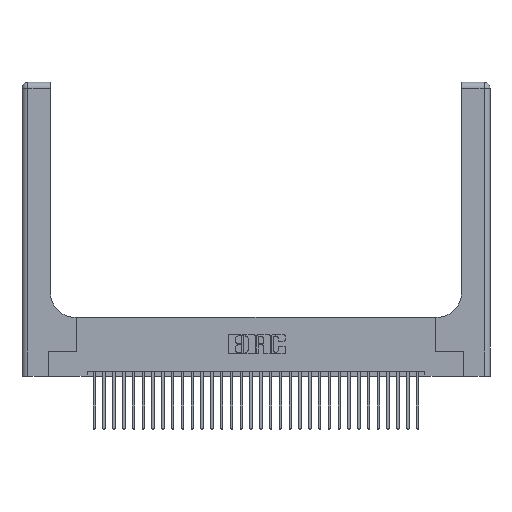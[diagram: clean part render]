
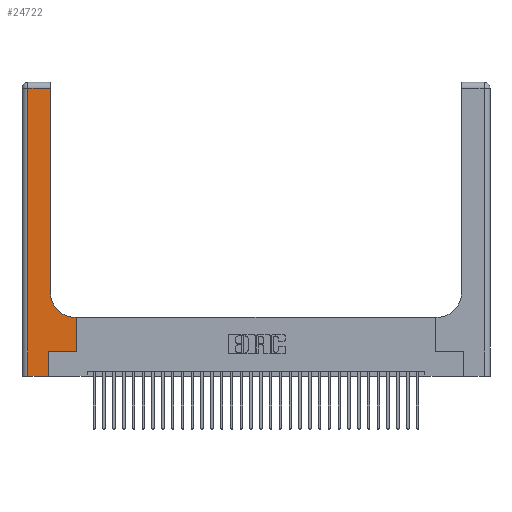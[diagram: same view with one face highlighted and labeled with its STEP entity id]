
A CAD part, top view. The second image highlights one B-rep face of the part: STEP entity #24722.
In plain terms, the highlighted planar face has unit normal (0, 0, 1).
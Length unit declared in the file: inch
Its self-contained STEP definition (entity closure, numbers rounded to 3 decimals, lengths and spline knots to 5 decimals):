
#365 = DIRECTION ( 'NONE',  ( -1., 0., 0. ) ) ;
#416 = VERTEX_POINT ( 'NONE', #21749 ) ;
#425 = EDGE_CURVE ( 'NONE', #14012, #24214, #13060, .T. ) ;
#596 = CARTESIAN_POINT ( 'NONE',  ( 0.5585, 0.25, 0.37 ) ) ;
#1376 = DIRECTION ( 'NONE',  ( -1., 0., 0. ) ) ;
#1511 = DIRECTION ( 'NONE',  ( 0., 1., 0. ) ) ;
#1523 = VERTEX_POINT ( 'NONE', #18330 ) ;
#1791 = VERTEX_POINT ( 'NONE', #2879 ) ;
#1811 = PLANE ( 'NONE',  #15789 ) ;
#2296 = VECTOR ( 'NONE', #27304, 39.37008 ) ;
#2879 = CARTESIAN_POINT ( 'NONE',  ( 0.269, 0., 0.37 ) ) ;
#2910 = EDGE_CURVE ( 'NONE', #24214, #5168, #25202, .T. ) ;
#3036 = FACE_OUTER_BOUND ( 'NONE', #20040, .T. ) ;
#3267 = CARTESIAN_POINT ( 'NONE',  ( 0.2915, 0.6, 0.37 ) ) ;
#4148 = CARTESIAN_POINT ( 'NONE',  ( 0., 3., 0.37 ) ) ;
#4423 = ORIENTED_EDGE ( 'NONE', *, *, #25913, .T. ) ;
#4759 = VECTOR ( 'NONE', #365, 39.37008 ) ;
#4827 = CARTESIAN_POINT ( 'NONE',  ( 0.06, 3., 0.37 ) ) ;
#5168 = VERTEX_POINT ( 'NONE', #31244 ) ;
#5522 = LINE ( 'NONE', #3267, #4759 ) ;
#6485 = CARTESIAN_POINT ( 'NONE',  ( 0.269, 0., 0.37 ) ) ;
#6946 = DIRECTION ( 'NONE',  ( 0., 0., -1. ) ) ;
#7225 = ORIENTED_EDGE ( 'NONE', *, *, #2910, .T. ) ;
#7393 = VECTOR ( 'NONE', #1511, 39.37008 ) ;
#7637 = CARTESIAN_POINT ( 'NONE',  ( 0., 0., 0.37 ) ) ;
#8522 = ORIENTED_EDGE ( 'NONE', *, *, #13523, .T. ) ;
#9076 = LINE ( 'NONE', #4827, #2296 ) ;
#9841 = LINE ( 'NONE', #21091, #22919 ) ;
#10006 = ORIENTED_EDGE ( 'NONE', *, *, #32723, .T. ) ;
#12406 = EDGE_CURVE ( 'NONE', #32494, #1523, #5522, .T. ) ;
#13060 = LINE ( 'NONE', #26183, #21402 ) ;
#13523 = EDGE_CURVE ( 'NONE', #5168, #26957, #9076, .T. ) ;
#14012 = VERTEX_POINT ( 'NONE', #28362 ) ;
#14065 = CARTESIAN_POINT ( 'NONE',  ( 0., 2.94, 0.37 ) ) ;
#14221 = DIRECTION ( 'NONE',  ( 1., 0., 0. ) ) ;
#15660 = CARTESIAN_POINT ( 'NONE',  ( 0.5585, 0.6, 0.37 ) ) ;
#15771 = VECTOR ( 'NONE', #23073, 39.37008 ) ;
#15789 = AXIS2_PLACEMENT_3D ( 'NONE', #4148, #32531, #19556 ) ;
#16133 = LINE ( 'NONE', #25100, #24888 ) ;
#16143 = ORIENTED_EDGE ( 'NONE', *, *, #12406, .T. ) ;
#16221 = DIRECTION ( 'NONE',  ( 0., 1., 0. ) ) ;
#17216 = EDGE_CURVE ( 'NONE', #20277, #32494, #9841, .T. ) ;
#17591 = CARTESIAN_POINT ( 'NONE',  ( 0.2915, 2.94, 0.37 ) ) ;
#17864 = EDGE_CURVE ( 'NONE', #416, #20277, #16133, .T. ) ;
#18121 = LINE ( 'NONE', #6485, #7393 ) ;
#18330 = CARTESIAN_POINT ( 'NONE',  ( 0.5415, 0.6, 0.37 ) ) ;
#19230 = VECTOR ( 'NONE', #1376, 39.37008 ) ;
#19556 = DIRECTION ( 'NONE',  ( -1., 0., 0. ) ) ;
#20040 = EDGE_LOOP ( 'NONE', ( #28948, #7225, #8522, #10006, #4423, #24714, #21469, #16143, #24076 ) ) ;
#20178 = EDGE_CURVE ( 'NONE', #1523, #14012, #21202, .T. ) ;
#20277 = VERTEX_POINT ( 'NONE', #596 ) ;
#21091 = CARTESIAN_POINT ( 'NONE',  ( 0.5585, 0.25, 0.37 ) ) ;
#21202 = CIRCLE ( 'NONE', #25435, 0.25 ) ;
#21402 = VECTOR ( 'NONE', #32028, 39.37008 ) ;
#21469 = ORIENTED_EDGE ( 'NONE', *, *, #17216, .T. ) ;
#21749 = CARTESIAN_POINT ( 'NONE',  ( 0.269, 0.25, 0.37 ) ) ;
#22180 = CARTESIAN_POINT ( 'NONE',  ( 0.5415, 0.85, 0.37 ) ) ;
#22919 = VECTOR ( 'NONE', #16221, 39.37008 ) ;
#23073 = DIRECTION ( 'NONE',  ( 1., 0., 0. ) ) ;
#24076 = ORIENTED_EDGE ( 'NONE', *, *, #20178, .T. ) ;
#24214 = VERTEX_POINT ( 'NONE', #17591 ) ;
#24714 = ORIENTED_EDGE ( 'NONE', *, *, #17864, .T. ) ;
#24722 = ADVANCED_FACE ( 'NONE', ( #3036 ), #1811, .F. ) ;
#24888 = VECTOR ( 'NONE', #27783, 39.37008 ) ;
#25100 = CARTESIAN_POINT ( 'NONE',  ( 0.269, 0.25, 0.37 ) ) ;
#25202 = LINE ( 'NONE', #14065, #19230 ) ;
#25435 = AXIS2_PLACEMENT_3D ( 'NONE', #22180, #6946, #14221 ) ;
#25913 = EDGE_CURVE ( 'NONE', #1791, #416, #18121, .T. ) ;
#26183 = CARTESIAN_POINT ( 'NONE',  ( 0.2915, 3., 0.37 ) ) ;
#26957 = VERTEX_POINT ( 'NONE', #31460 ) ;
#27304 = DIRECTION ( 'NONE',  ( 0., -1., 0. ) ) ;
#27783 = DIRECTION ( 'NONE',  ( 1., 0., 0. ) ) ;
#28362 = CARTESIAN_POINT ( 'NONE',  ( 0.2915, 0.85, 0.37 ) ) ;
#28948 = ORIENTED_EDGE ( 'NONE', *, *, #425, .T. ) ;
#30547 = LINE ( 'NONE', #7637, #15771 ) ;
#31244 = CARTESIAN_POINT ( 'NONE',  ( 0.06, 2.94, 0.37 ) ) ;
#31460 = CARTESIAN_POINT ( 'NONE',  ( 0.06, 0., 0.37 ) ) ;
#32028 = DIRECTION ( 'NONE',  ( 0., 1., 0. ) ) ;
#32494 = VERTEX_POINT ( 'NONE', #15660 ) ;
#32531 = DIRECTION ( 'NONE',  ( 0., 0., -1. ) ) ;
#32723 = EDGE_CURVE ( 'NONE', #26957, #1791, #30547, .T. ) ;
